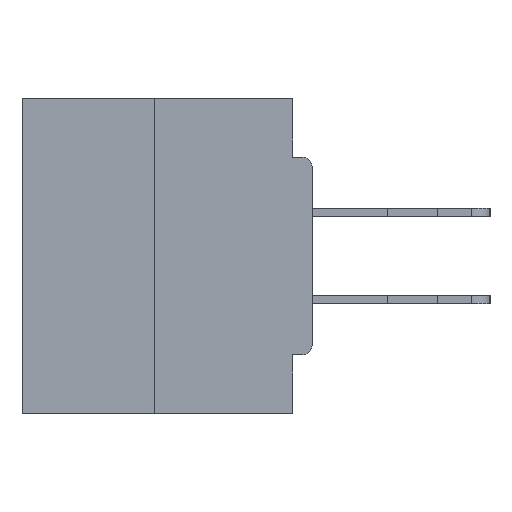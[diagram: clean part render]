
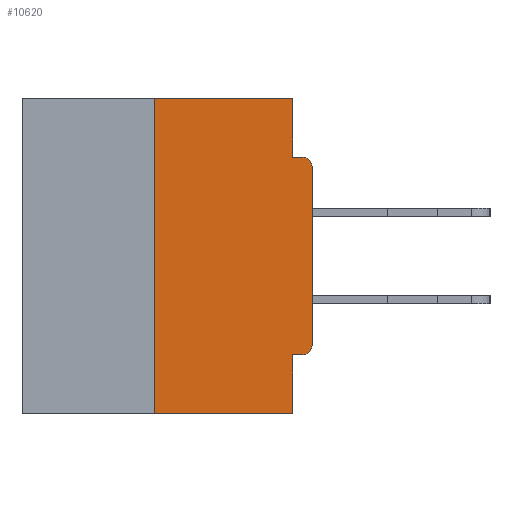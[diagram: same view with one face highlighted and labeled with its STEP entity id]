
A CAD part, left-side view. The second image highlights one B-rep face of the part: STEP entity #10620.
In plain terms, the highlighted planar face has unit normal (-1, 0, 0).
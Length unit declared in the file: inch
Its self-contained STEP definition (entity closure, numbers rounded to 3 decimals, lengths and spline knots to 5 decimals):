
#314 = DIRECTION ( 'NONE',  ( 0., 0., -1. ) ) ;
#610 = ORIENTED_EDGE ( 'NONE', *, *, #6360, .T. ) ;
#685 = LINE ( 'NONE', #5528, #29767 ) ;
#1969 = LINE ( 'NONE', #9703, #30266 ) ;
#2116 = VERTEX_POINT ( 'NONE', #28065 ) ;
#2366 = EDGE_CURVE ( 'NONE', #13606, #2116, #32245, .T. ) ;
#2401 = EDGE_CURVE ( 'NONE', #28572, #13606, #11482, .T. ) ;
#2907 = VERTEX_POINT ( 'NONE', #21756 ) ;
#3445 = LINE ( 'NONE', #4054, #6229 ) ;
#3785 = VERTEX_POINT ( 'NONE', #31405 ) ;
#4054 = CARTESIAN_POINT ( 'NONE',  ( 0., 0.031, 0. ) ) ;
#4133 = ORIENTED_EDGE ( 'NONE', *, *, #2401, .F. ) ;
#4571 = CARTESIAN_POINT ( 'NONE',  ( 0., 0., 0. ) ) ;
#4715 = VECTOR ( 'NONE', #30275, 39.37008 ) ;
#5012 = DIRECTION ( 'NONE',  ( 0., -1., 0. ) ) ;
#5513 = DIRECTION ( 'NONE',  ( 0., 0., -1. ) ) ;
#5528 = CARTESIAN_POINT ( 'NONE',  ( 0., 0.031, -0.5 ) ) ;
#5707 = EDGE_CURVE ( 'NONE', #28572, #2907, #17091, .T. ) ;
#6098 = DIRECTION ( 'NONE',  ( -1., 0., 0. ) ) ;
#6229 = VECTOR ( 'NONE', #19093, 39.37008 ) ;
#6360 = EDGE_CURVE ( 'NONE', #3785, #18579, #13487, .T. ) ;
#6803 = DIRECTION ( 'NONE',  ( 0., 1., 0. ) ) ;
#7210 = PLANE ( 'NONE',  #27423 ) ;
#7507 = EDGE_CURVE ( 'NONE', #29393, #2907, #685, .T. ) ;
#8114 = CARTESIAN_POINT ( 'NONE',  ( 0., 0.031, -0.0935 ) ) ;
#8176 = DIRECTION ( 'NONE',  ( -1., 0., 0. ) ) ;
#9234 = CARTESIAN_POINT ( 'NONE',  ( 0., 0.46, -0.5 ) ) ;
#9479 = CARTESIAN_POINT ( 'NONE',  ( 0., 0.015, -0.0935 ) ) ;
#9628 = ORIENTED_EDGE ( 'NONE', *, *, #5707, .T. ) ;
#9703 = CARTESIAN_POINT ( 'NONE',  ( 0., 0., -0.4065 ) ) ;
#9867 = VECTOR ( 'NONE', #12623, 39.37008 ) ;
#10369 = AXIS2_PLACEMENT_3D ( 'NONE', #20773, #8176, #5513 ) ;
#10620 = ADVANCED_FACE ( 'NONE', ( #25131 ), #7210, .F. ) ;
#11304 = EDGE_CURVE ( 'NONE', #2116, #11650, #3445, .T. ) ;
#11482 = LINE ( 'NONE', #30487, #4715 ) ;
#11650 = VERTEX_POINT ( 'NONE', #8114 ) ;
#11904 = DIRECTION ( 'NONE',  ( 0., 0., 1. ) ) ;
#12205 = CARTESIAN_POINT ( 'NONE',  ( 0., 0.015, -0.4065 ) ) ;
#12328 = CARTESIAN_POINT ( 'NONE',  ( 0., 0.46, 0. ) ) ;
#12539 = DIRECTION ( 'NONE',  ( 0., 0., -1. ) ) ;
#12618 = EDGE_CURVE ( 'NONE', #22226, #22543, #23657, .T. ) ;
#12623 = DIRECTION ( 'NONE',  ( 0., -1., 0. ) ) ;
#13457 = CARTESIAN_POINT ( 'NONE',  ( 0., 0.015, -0.1085 ) ) ;
#13487 = CIRCLE ( 'NONE', #29023, 0.015 ) ;
#13606 = VERTEX_POINT ( 'NONE', #15082 ) ;
#13689 = DIRECTION ( 'NONE',  ( 0., 0., -1. ) ) ;
#15014 = CARTESIAN_POINT ( 'NONE',  ( 0., 0., -0.0935 ) ) ;
#15082 = CARTESIAN_POINT ( 'NONE',  ( 0., 0.25, 0. ) ) ;
#15613 = EDGE_CURVE ( 'NONE', #11650, #18579, #16758, .T. ) ;
#15880 = LINE ( 'NONE', #4571, #30242 ) ;
#16386 = EDGE_CURVE ( 'NONE', #22543, #3785, #15880, .T. ) ;
#16758 = LINE ( 'NONE', #15014, #31882 ) ;
#17091 = LINE ( 'NONE', #9234, #31028 ) ;
#17100 = ORIENTED_EDGE ( 'NONE', *, *, #26986, .F. ) ;
#17438 = CARTESIAN_POINT ( 'NONE',  ( 0., 0.031, -0.4065 ) ) ;
#17504 = ORIENTED_EDGE ( 'NONE', *, *, #7507, .F. ) ;
#18579 = VERTEX_POINT ( 'NONE', #9479 ) ;
#19093 = DIRECTION ( 'NONE',  ( 0., 0., -1. ) ) ;
#19331 = CARTESIAN_POINT ( 'NONE',  ( 0., 0., -0.3915 ) ) ;
#19784 = DIRECTION ( 'NONE',  ( 0., -1., 0. ) ) ;
#20773 = CARTESIAN_POINT ( 'NONE',  ( 0., 0.015, -0.3915 ) ) ;
#21756 = CARTESIAN_POINT ( 'NONE',  ( 0., 0.031, -0.5 ) ) ;
#22226 = VERTEX_POINT ( 'NONE', #12205 ) ;
#22337 = ORIENTED_EDGE ( 'NONE', *, *, #12618, .T. ) ;
#22543 = VERTEX_POINT ( 'NONE', #19331 ) ;
#23657 = CIRCLE ( 'NONE', #10369, 0.015 ) ;
#24638 = ORIENTED_EDGE ( 'NONE', *, *, #15613, .F. ) ;
#25131 = FACE_OUTER_BOUND ( 'NONE', #27899, .T. ) ;
#26986 = EDGE_CURVE ( 'NONE', #22226, #29393, #1969, .T. ) ;
#27182 = ORIENTED_EDGE ( 'NONE', *, *, #16386, .T. ) ;
#27423 = AXIS2_PLACEMENT_3D ( 'NONE', #12328, #27810, #12539 ) ;
#27560 = ORIENTED_EDGE ( 'NONE', *, *, #11304, .F. ) ;
#27810 = DIRECTION ( 'NONE',  ( 1., 0., 0. ) ) ;
#27899 = EDGE_LOOP ( 'NONE', ( #32340, #4133, #9628, #17504, #17100, #22337, #27182, #610, #24638, #27560 ) ) ;
#28065 = CARTESIAN_POINT ( 'NONE',  ( 0., 0.031, 0. ) ) ;
#28572 = VERTEX_POINT ( 'NONE', #30892 ) ;
#29023 = AXIS2_PLACEMENT_3D ( 'NONE', #13457, #6098, #13689 ) ;
#29393 = VERTEX_POINT ( 'NONE', #17438 ) ;
#29603 = CARTESIAN_POINT ( 'NONE',  ( 0., 0.46, 0. ) ) ;
#29767 = VECTOR ( 'NONE', #314, 39.37008 ) ;
#30242 = VECTOR ( 'NONE', #11904, 39.37008 ) ;
#30266 = VECTOR ( 'NONE', #6803, 39.37008 ) ;
#30275 = DIRECTION ( 'NONE',  ( 0., 0., 1. ) ) ;
#30487 = CARTESIAN_POINT ( 'NONE',  ( 0., 0.25, 0. ) ) ;
#30892 = CARTESIAN_POINT ( 'NONE',  ( 0., 0.25, -0.5 ) ) ;
#31028 = VECTOR ( 'NONE', #5012, 39.37008 ) ;
#31405 = CARTESIAN_POINT ( 'NONE',  ( 0., 0., -0.1085 ) ) ;
#31882 = VECTOR ( 'NONE', #19784, 39.37008 ) ;
#32245 = LINE ( 'NONE', #29603, #9867 ) ;
#32340 = ORIENTED_EDGE ( 'NONE', *, *, #2366, .F. ) ;
